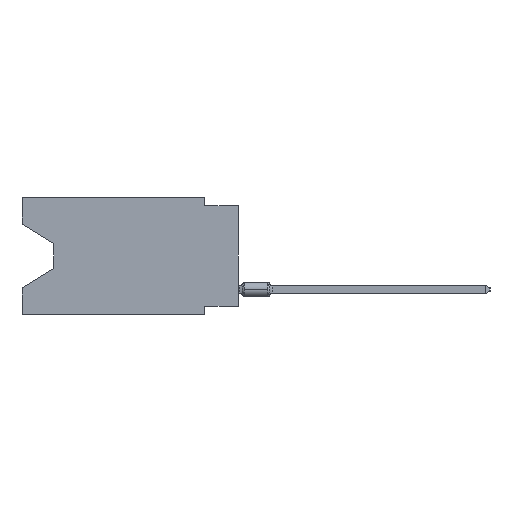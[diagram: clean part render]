
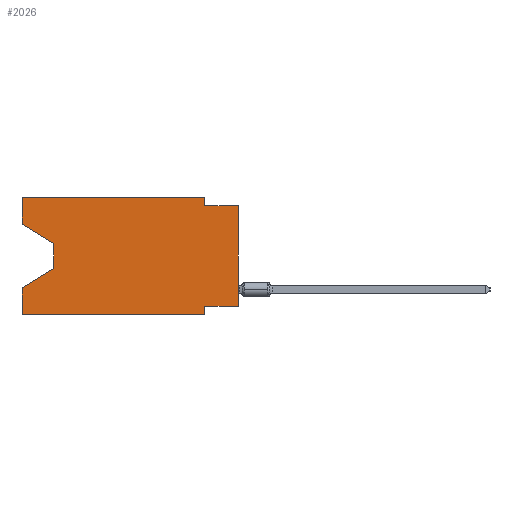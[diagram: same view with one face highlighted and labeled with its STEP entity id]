
A CAD part, left-side view. The second image highlights one B-rep face of the part: STEP entity #2026.
In plain terms, the highlighted planar face has unit normal (-1, 0, 0).
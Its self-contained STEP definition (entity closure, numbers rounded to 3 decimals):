
#2026 = ADVANCED_FACE ( 'NONE', ( #63900 ), #19223, .F. ) ;
#3226 = ORIENTED_EDGE ( 'NONE', *, *, #98604, .F. ) ;
#6158 = LINE ( 'NONE', #22694, #74319 ) ;
#7652 = EDGE_CURVE ( 'NONE', #27048, #52072, #40505, .T. ) ;
#11620 = ORIENTED_EDGE ( 'NONE', *, *, #47773, .F. ) ;
#12493 = LINE ( 'NONE', #84224, #69781 ) ;
#12572 = ORIENTED_EDGE ( 'NONE', *, *, #85921, .F. ) ;
#14949 = LINE ( 'NONE', #86672, #24558 ) ;
#16802 = DIRECTION ( 'NONE',  ( 0., 0., 1. ) ) ;
#16958 = CARTESIAN_POINT ( 'NONE',  ( 0., 13.97, -5.385 ) ) ;
#17062 = ORIENTED_EDGE ( 'NONE', *, *, #113174, .F. ) ;
#18316 = LINE ( 'NONE', #90055, #116173 ) ;
#19223 = PLANE ( 'NONE',  #103998 ) ;
#19863 = DIRECTION ( 'NONE',  ( 0., 0., 1. ) ) ;
#20708 = EDGE_CURVE ( 'NONE', #45033, #75697, #22109, .T. ) ;
#22109 = LINE ( 'NONE', #29223, #86578 ) ;
#22694 = CARTESIAN_POINT ( 'NONE',  ( 0., 2.54, -8.89 ) ) ;
#24558 = VECTOR ( 'NONE', #67859, 1000. ) ;
#27048 = VERTEX_POINT ( 'NONE', #69182 ) ;
#28953 = CARTESIAN_POINT ( 'NONE',  ( 0., 16.383, 0. ) ) ;
#29223 = CARTESIAN_POINT ( 'NONE',  ( 0., 16.383, -8.89 ) ) ;
#29867 = DIRECTION ( 'NONE',  ( 0., 0., -1. ) ) ;
#34315 = VECTOR ( 'NONE', #16802, 1000. ) ;
#35052 = EDGE_CURVE ( 'NONE', #36174, #40590, #101654, .T. ) ;
#35634 = CARTESIAN_POINT ( 'NONE',  ( 0., 16.383, 0. ) ) ;
#36174 = VERTEX_POINT ( 'NONE', #28953 ) ;
#38858 = ORIENTED_EDGE ( 'NONE', *, *, #92908, .T. ) ;
#39785 = DIRECTION ( 'NONE',  ( 0., 0., -1. ) ) ;
#40496 = DIRECTION ( 'NONE',  ( 0., -1., 0. ) ) ;
#40505 = LINE ( 'NONE', #112217, #73063 ) ;
#40590 = VERTEX_POINT ( 'NONE', #70509 ) ;
#41721 = CARTESIAN_POINT ( 'NONE',  ( 0., 16.383, -6.852 ) ) ;
#43581 = ORIENTED_EDGE ( 'NONE', *, *, #7652, .F. ) ;
#45033 = VERTEX_POINT ( 'NONE', #93843 ) ;
#46283 = ORIENTED_EDGE ( 'NONE', *, *, #20708, .T. ) ;
#47639 = EDGE_LOOP ( 'NONE', ( #91807, #109247, #38858, #68106, #46283, #11620, #12572, #51924, #43581, #3226, #105853, #17062 ) ) ;
#47773 = EDGE_CURVE ( 'NONE', #61296, #75697, #6158, .T. ) ;
#49196 = CARTESIAN_POINT ( 'NONE',  ( 0., 0., -8.255 ) ) ;
#49980 = VECTOR ( 'NONE', #115765, 1000. ) ;
#51924 = ORIENTED_EDGE ( 'NONE', *, *, #62014, .T. ) ;
#52072 = VERTEX_POINT ( 'NONE', #96253 ) ;
#53071 = EDGE_CURVE ( 'NONE', #102858, #99826, #18316, .T. ) ;
#54089 = VERTEX_POINT ( 'NONE', #107808 ) ;
#56754 = VECTOR ( 'NONE', #19863, 1000. ) ;
#57577 = EDGE_CURVE ( 'NONE', #45033, #113730, #97367, .T. ) ;
#57973 = CARTESIAN_POINT ( 'NONE',  ( 0., 16.383, 0. ) ) ;
#59573 = VECTOR ( 'NONE', #104614, 1000. ) ;
#61296 = VERTEX_POINT ( 'NONE', #92012 ) ;
#62014 = EDGE_CURVE ( 'NONE', #109954, #52072, #107503, .T. ) ;
#63900 = FACE_OUTER_BOUND ( 'NONE', #47639, .T. ) ;
#66563 = DIRECTION ( 'NONE',  ( 0., 0., 1. ) ) ;
#67859 = DIRECTION ( 'NONE',  ( 0., 0., -1. ) ) ;
#67882 = CARTESIAN_POINT ( 'NONE',  ( 0., 13.97, -3.505 ) ) ;
#67967 = CARTESIAN_POINT ( 'NONE',  ( 0., 2.54, -8.89 ) ) ;
#68106 = ORIENTED_EDGE ( 'NONE', *, *, #57577, .F. ) ;
#68715 = LINE ( 'NONE', #16958, #59573 ) ;
#69182 = CARTESIAN_POINT ( 'NONE',  ( 0., 2.54, -0.635 ) ) ;
#69781 = VECTOR ( 'NONE', #66563, 1000. ) ;
#70509 = CARTESIAN_POINT ( 'NONE',  ( 0., 2.54, 0. ) ) ;
#72594 = VECTOR ( 'NONE', #29867, 1000. ) ;
#73063 = VECTOR ( 'NONE', #94571, 1000. ) ;
#74319 = VECTOR ( 'NONE', #102660, 1000. ) ;
#75125 = LINE ( 'NONE', #83929, #72594 ) ;
#75639 = DIRECTION ( 'NONE',  ( 1., 0., 0. ) ) ;
#75697 = VERTEX_POINT ( 'NONE', #67967 ) ;
#83929 = CARTESIAN_POINT ( 'NONE',  ( 0., 13.97, -3.505 ) ) ;
#84224 = CARTESIAN_POINT ( 'NONE',  ( 0., 16.383, 0. ) ) ;
#85921 = EDGE_CURVE ( 'NONE', #109954, #61296, #115191, .T. ) ;
#86578 = VECTOR ( 'NONE', #100935, 1000. ) ;
#86672 = CARTESIAN_POINT ( 'NONE',  ( 0., 2.54, 0. ) ) ;
#90055 = CARTESIAN_POINT ( 'NONE',  ( 0., 16.383, -2.038 ) ) ;
#90637 = DIRECTION ( 'NONE',  ( 0., -0.855, -0.519 ) ) ;
#91807 = ORIENTED_EDGE ( 'NONE', *, *, #53071, .T. ) ;
#91963 = EDGE_CURVE ( 'NONE', #99826, #54089, #75125, .T. ) ;
#92012 = CARTESIAN_POINT ( 'NONE',  ( 0., 2.54, -8.255 ) ) ;
#92908 = EDGE_CURVE ( 'NONE', #54089, #113730, #68715, .T. ) ;
#93843 = CARTESIAN_POINT ( 'NONE',  ( 0., 16.383, -8.89 ) ) ;
#94571 = DIRECTION ( 'NONE',  ( 0., -1., 0. ) ) ;
#96253 = CARTESIAN_POINT ( 'NONE',  ( 0., 0., -0.635 ) ) ;
#97367 = LINE ( 'NONE', #35634, #34315 ) ;
#98604 = EDGE_CURVE ( 'NONE', #40590, #27048, #14949, .T. ) ;
#99826 = VERTEX_POINT ( 'NONE', #67882 ) ;
#100432 = CARTESIAN_POINT ( 'NONE',  ( 0., 0., 0. ) ) ;
#100502 = CARTESIAN_POINT ( 'NONE',  ( 0., 16.383, 0. ) ) ;
#100935 = DIRECTION ( 'NONE',  ( 0., -1., 0. ) ) ;
#101075 = VECTOR ( 'NONE', #40496, 1000. ) ;
#101654 = LINE ( 'NONE', #100502, #101075 ) ;
#102660 = DIRECTION ( 'NONE',  ( 0., 0., -1. ) ) ;
#102858 = VERTEX_POINT ( 'NONE', #112751 ) ;
#103998 = AXIS2_PLACEMENT_3D ( 'NONE', #57973, #75639, #39785 ) ;
#104614 = DIRECTION ( 'NONE',  ( 0., 0.855, -0.519 ) ) ;
#105853 = ORIENTED_EDGE ( 'NONE', *, *, #35052, .F. ) ;
#107503 = LINE ( 'NONE', #100432, #56754 ) ;
#107808 = CARTESIAN_POINT ( 'NONE',  ( 0., 13.97, -5.385 ) ) ;
#108125 = CARTESIAN_POINT ( 'NONE',  ( 0., 0., -8.255 ) ) ;
#109247 = ORIENTED_EDGE ( 'NONE', *, *, #91963, .T. ) ;
#109954 = VERTEX_POINT ( 'NONE', #49196 ) ;
#112217 = CARTESIAN_POINT ( 'NONE',  ( 0., 0., -0.635 ) ) ;
#112751 = CARTESIAN_POINT ( 'NONE',  ( 0., 16.383, -2.038 ) ) ;
#113174 = EDGE_CURVE ( 'NONE', #102858, #36174, #12493, .T. ) ;
#113730 = VERTEX_POINT ( 'NONE', #41721 ) ;
#115191 = LINE ( 'NONE', #108125, #49980 ) ;
#115765 = DIRECTION ( 'NONE',  ( 0., 1., 0. ) ) ;
#116173 = VECTOR ( 'NONE', #90637, 1000. ) ;
